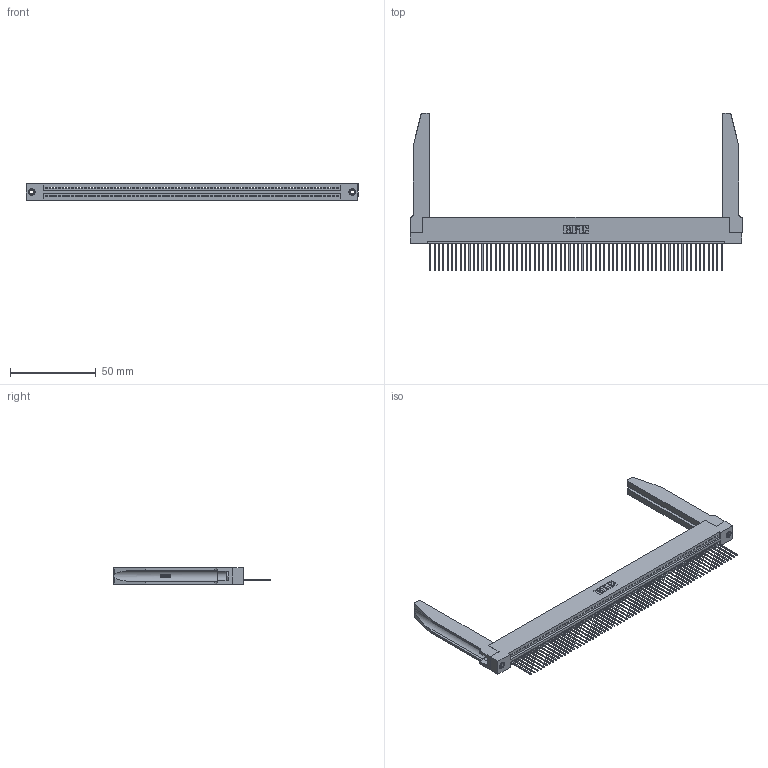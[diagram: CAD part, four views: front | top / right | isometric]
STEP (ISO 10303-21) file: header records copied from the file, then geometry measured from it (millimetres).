
FILE_DESCRIPTION (( 'STEP AP203' ), '1' );
FILE_NAME ('345-068-542-178.STEP', '2019-10-12T07:15:52', ( '' ), ( '' ), 'SwSTEP 2.0', 'SolidWorks 2016', '' );
FILE_SCHEMA (( 'CONFIG_CONTROL_DESIGN' ));
Length unit declared in the file: inch
Products named in the file (5): 345-220-078_345-220-078; 345-068-542-178; 345 Part_Flush Mounting Lugs - 0.156 Dia-TH; 345-292-001_345-293-142; 345-250-001_345-250-001-102
Assembly tree (73 placements, depth 2):
  345-068-542-178
    345 Part_Flush Mounting Lugs - 0.156 Dia-TH
    345-292-001_345-293-142  x68
    345-250-001_345-250-001-102  x2
    345-220-078_345-220-078  x2
Bounding box: 193.95 x 92.25 x 9.4 mm (x, y, z)
Volume: 26556.7 mm3; surface area: 33121 mm2
Topology: 73 solids, 73 shells, 4304 faces, 12917 edges, 8510 vertices
Faces by surface type: plane 2942, cylinder 1310, bspline 36, cone 12, torus 4
Entity records: 52436 total; most frequent: CARTESIAN_POINT 9979, ORIENTED_EDGE 8878, DIRECTION 7685, EDGE_CURVE 4439, LINE 3941, VECTOR 3941, VERTEX_POINT 2952, AXIS2_PLACEMENT_3D 1872
